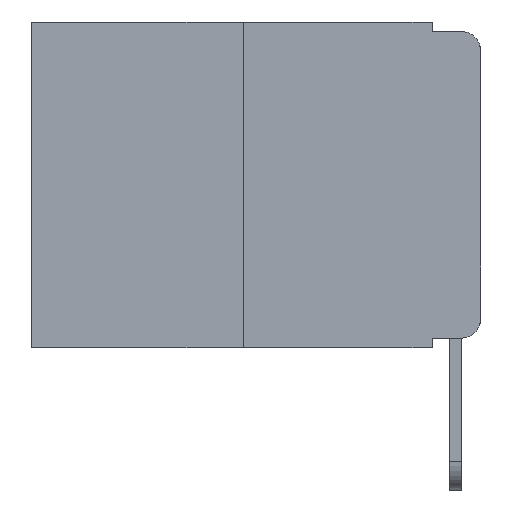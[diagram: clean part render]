
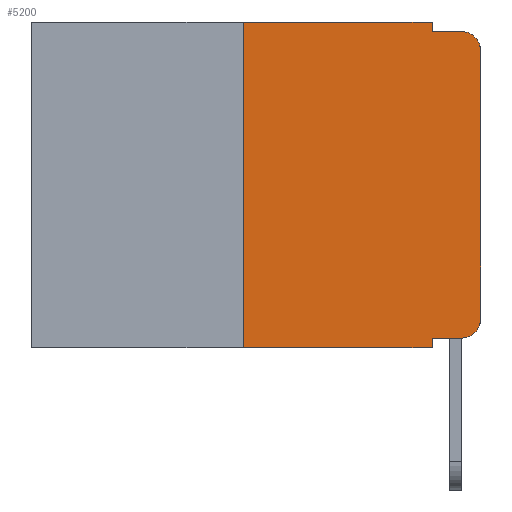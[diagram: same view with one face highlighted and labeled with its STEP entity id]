
A CAD part, left-side view. The second image highlights one B-rep face of the part: STEP entity #5200.
In plain terms, the highlighted planar face has unit normal (-1, 0, 0).
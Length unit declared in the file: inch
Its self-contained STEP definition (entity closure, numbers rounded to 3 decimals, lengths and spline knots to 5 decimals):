
#30 = VECTOR ( 'NONE', #20782, 39.37008 ) ;
#610 = CARTESIAN_POINT ( 'NONE',  ( 0., 0.25, 0. ) ) ;
#1017 = VERTEX_POINT ( 'NONE', #16024 ) ;
#1602 = DIRECTION ( 'NONE',  ( 0., 0., -1. ) ) ;
#2033 = DIRECTION ( 'NONE',  ( 0., 0., 1. ) ) ;
#2063 = EDGE_LOOP ( 'NONE', ( #13790, #14503, #8201, #2482, #11627, #8968, #18636, #13374, #14507, #4860 ) ) ;
#2482 = ORIENTED_EDGE ( 'NONE', *, *, #7995, .F. ) ;
#2531 = DIRECTION ( 'NONE',  ( 0., 0., 1. ) ) ;
#2641 = DIRECTION ( 'NONE',  ( 1., 0., 0. ) ) ;
#3399 = CARTESIAN_POINT ( 'NONE',  ( 0., 0.051, -0.01 ) ) ;
#3507 = LINE ( 'NONE', #11806, #20225 ) ;
#3519 = EDGE_CURVE ( 'NONE', #3587, #14894, #15204, .T. ) ;
#3587 = VERTEX_POINT ( 'NONE', #18696 ) ;
#3730 = AXIS2_PLACEMENT_3D ( 'NONE', #20596, #11460, #1602 ) ;
#3949 = CARTESIAN_POINT ( 'NONE',  ( 0., 0.051, 0. ) ) ;
#4668 = EDGE_CURVE ( 'NONE', #18383, #3587, #6054, .T. ) ;
#4860 = ORIENTED_EDGE ( 'NONE', *, *, #3519, .T. ) ;
#5046 = DIRECTION ( 'NONE',  ( 0., 0., -1. ) ) ;
#5185 = VERTEX_POINT ( 'NONE', #19940 ) ;
#5200 = ADVANCED_FACE ( 'NONE', ( #13145 ), #10741, .F. ) ;
#5515 = CARTESIAN_POINT ( 'NONE',  ( 0., 0.051, -0.333 ) ) ;
#5644 = VERTEX_POINT ( 'NONE', #14260 ) ;
#5785 = EDGE_CURVE ( 'NONE', #18383, #12105, #20085, .T. ) ;
#5948 = CARTESIAN_POINT ( 'NONE',  ( 0., 0.473, 0. ) ) ;
#5995 = CARTESIAN_POINT ( 'NONE',  ( 0., 0.051, -0.01 ) ) ;
#6054 = LINE ( 'NONE', #12531, #9786 ) ;
#6158 = DIRECTION ( 'NONE',  ( -1., 0., 0. ) ) ;
#6441 = VECTOR ( 'NONE', #2531, 39.37008 ) ;
#6570 = LINE ( 'NONE', #5995, #10284 ) ;
#6890 = EDGE_CURVE ( 'NONE', #1017, #5185, #18869, .T. ) ;
#7594 = DIRECTION ( 'NONE',  ( 0., -1., 0. ) ) ;
#7995 = EDGE_CURVE ( 'NONE', #15703, #12068, #12027, .T. ) ;
#8054 = CIRCLE ( 'NONE', #3730, 0.02 ) ;
#8201 = ORIENTED_EDGE ( 'NONE', *, *, #9039, .F. ) ;
#8659 = VECTOR ( 'NONE', #13122, 39.37008 ) ;
#8968 = ORIENTED_EDGE ( 'NONE', *, *, #6890, .F. ) ;
#9039 = EDGE_CURVE ( 'NONE', #12068, #16651, #6570, .T. ) ;
#9151 = LINE ( 'NONE', #14597, #8659 ) ;
#9786 = VECTOR ( 'NONE', #20161, 39.37008 ) ;
#10058 = EDGE_CURVE ( 'NONE', #5644, #16651, #8054, .T. ) ;
#10284 = VECTOR ( 'NONE', #7594, 39.37008 ) ;
#10741 = PLANE ( 'NONE',  #11654 ) ;
#11460 = DIRECTION ( 'NONE',  ( -1., 0., 0. ) ) ;
#11627 = ORIENTED_EDGE ( 'NONE', *, *, #18232, .F. ) ;
#11654 = AXIS2_PLACEMENT_3D ( 'NONE', #5948, #2641, #13880 ) ;
#11806 = CARTESIAN_POINT ( 'NONE',  ( 0., 0., 0. ) ) ;
#11982 = DIRECTION ( 'NONE',  ( 0., 0., -1. ) ) ;
#12027 = LINE ( 'NONE', #3949, #19686 ) ;
#12068 = VERTEX_POINT ( 'NONE', #3399 ) ;
#12105 = VERTEX_POINT ( 'NONE', #16205 ) ;
#12185 = EDGE_CURVE ( 'NONE', #14894, #5644, #3507, .T. ) ;
#12322 = LINE ( 'NONE', #14687, #30 ) ;
#12531 = CARTESIAN_POINT ( 'NONE',  ( 0., 0.051, -0.333 ) ) ;
#12914 = CARTESIAN_POINT ( 'NONE',  ( 0., 0., -0.313 ) ) ;
#13122 = DIRECTION ( 'NONE',  ( 0., -1., 0. ) ) ;
#13145 = FACE_OUTER_BOUND ( 'NONE', #2063, .T. ) ;
#13374 = ORIENTED_EDGE ( 'NONE', *, *, #5785, .F. ) ;
#13675 = CARTESIAN_POINT ( 'NONE',  ( 0., 0.02, -0.01 ) ) ;
#13790 = ORIENTED_EDGE ( 'NONE', *, *, #12185, .T. ) ;
#13880 = DIRECTION ( 'NONE',  ( 0., 0., -1. ) ) ;
#14260 = CARTESIAN_POINT ( 'NONE',  ( 0., 0., -0.03 ) ) ;
#14503 = ORIENTED_EDGE ( 'NONE', *, *, #10058, .T. ) ;
#14507 = ORIENTED_EDGE ( 'NONE', *, *, #4668, .T. ) ;
#14597 = CARTESIAN_POINT ( 'NONE',  ( 0., 0.473, -0.343 ) ) ;
#14687 = CARTESIAN_POINT ( 'NONE',  ( 0., 0.473, 0. ) ) ;
#14894 = VERTEX_POINT ( 'NONE', #12914 ) ;
#15204 = CIRCLE ( 'NONE', #19459, 0.02 ) ;
#15574 = CARTESIAN_POINT ( 'NONE',  ( 0., 0.02, -0.313 ) ) ;
#15703 = VERTEX_POINT ( 'NONE', #15934 ) ;
#15934 = CARTESIAN_POINT ( 'NONE',  ( 0., 0.051, 0. ) ) ;
#16024 = CARTESIAN_POINT ( 'NONE',  ( 0., 0.25, -0.343 ) ) ;
#16054 = VECTOR ( 'NONE', #5046, 39.37008 ) ;
#16205 = CARTESIAN_POINT ( 'NONE',  ( 0., 0.051, -0.343 ) ) ;
#16651 = VERTEX_POINT ( 'NONE', #13675 ) ;
#17073 = DIRECTION ( 'NONE',  ( 0., 0., -1. ) ) ;
#17568 = CARTESIAN_POINT ( 'NONE',  ( 0., 0.051, 0. ) ) ;
#18232 = EDGE_CURVE ( 'NONE', #5185, #15703, #12322, .T. ) ;
#18383 = VERTEX_POINT ( 'NONE', #5515 ) ;
#18636 = ORIENTED_EDGE ( 'NONE', *, *, #18981, .T. ) ;
#18696 = CARTESIAN_POINT ( 'NONE',  ( 0., 0.02, -0.333 ) ) ;
#18869 = LINE ( 'NONE', #610, #6441 ) ;
#18981 = EDGE_CURVE ( 'NONE', #1017, #12105, #9151, .T. ) ;
#19459 = AXIS2_PLACEMENT_3D ( 'NONE', #15574, #6158, #17073 ) ;
#19686 = VECTOR ( 'NONE', #11982, 39.37008 ) ;
#19940 = CARTESIAN_POINT ( 'NONE',  ( 0., 0.25, 0. ) ) ;
#20085 = LINE ( 'NONE', #17568, #16054 ) ;
#20161 = DIRECTION ( 'NONE',  ( 0., -1., 0. ) ) ;
#20225 = VECTOR ( 'NONE', #2033, 39.37008 ) ;
#20596 = CARTESIAN_POINT ( 'NONE',  ( 0., 0.02, -0.03 ) ) ;
#20782 = DIRECTION ( 'NONE',  ( 0., -1., 0. ) ) ;
